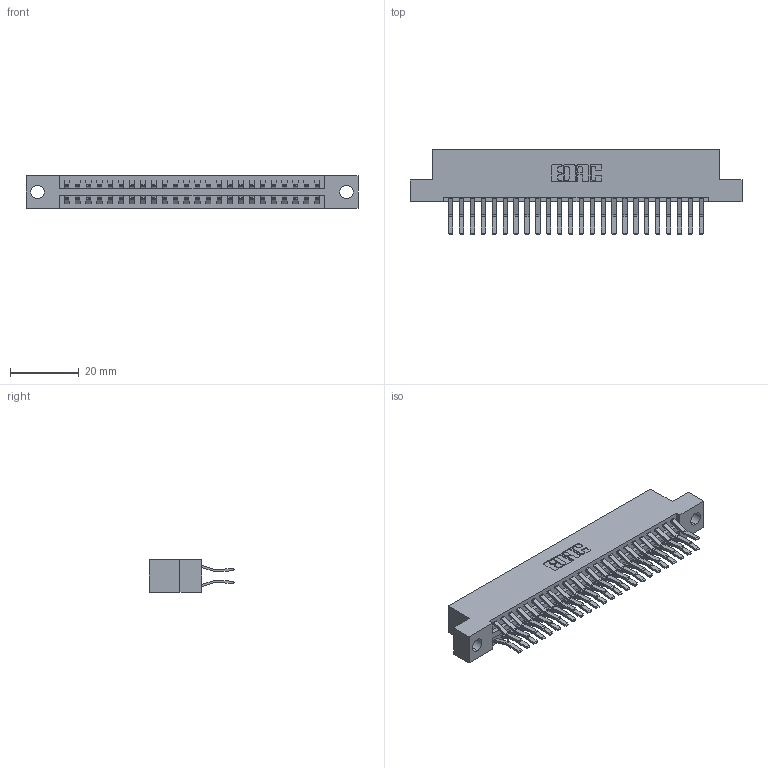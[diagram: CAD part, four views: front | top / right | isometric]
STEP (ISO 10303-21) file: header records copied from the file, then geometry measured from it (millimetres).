
FILE_DESCRIPTION (( 'STEP AP203' ), '1' );
FILE_NAME ('396-048-560-204.STEP', '2018-09-08T01:25:20', ( '' ), ( '' ), 'SwSTEP 2.0', 'SolidWorks 2016', '' );
FILE_SCHEMA (( 'CONFIG_CONTROL_DESIGN' ));
Length unit declared in the file: inch
Products named in the file (3): 345-292-001_560 Tail; 396-048-560-204; 346 Part_Flush Mounting Lugs - 0.156 Dia-TH
Assembly tree (49 placements, depth 2):
  396-048-560-204
    346 Part_Flush Mounting Lugs - 0.156 Dia-TH
    345-292-001_560 Tail  x48
Bounding box: 96.77 x 24.78 x 9.4 mm (x, y, z)
Volume: 9523.6 mm3; surface area: 13460.7 mm2
Topology: 49 solids, 49 shells, 2714 faces, 8057 edges, 5306 vertices
Faces by surface type: plane 1756, cylinder 958
Entity records: 18177 total; most frequent: CARTESIAN_POINT 3020, ORIENTED_EDGE 2954, DIRECTION 2717, EDGE_CURVE 1477, VECTOR 1245, LINE 1245, VERTEX_POINT 982, AXIS2_PLACEMENT_3D 736
